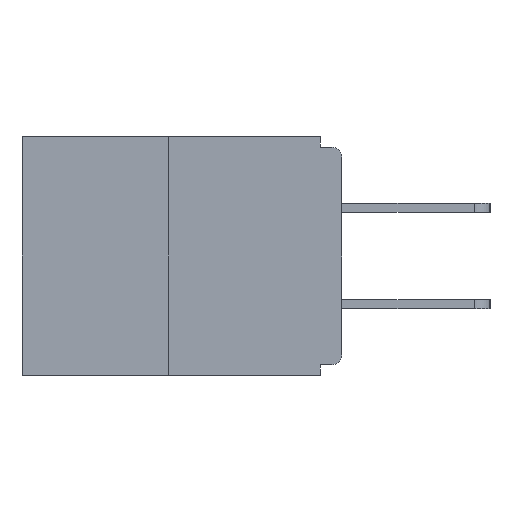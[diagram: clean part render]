
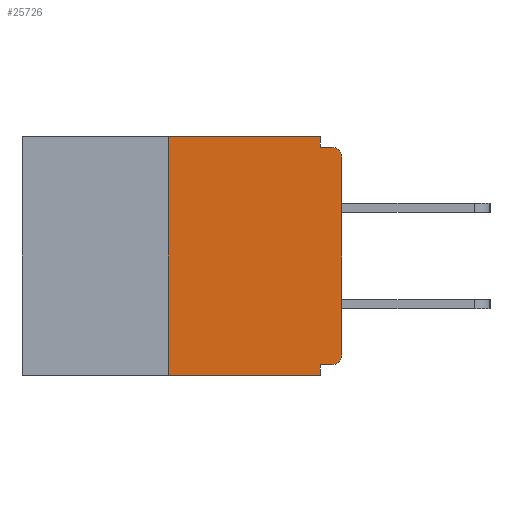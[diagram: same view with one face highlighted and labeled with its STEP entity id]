
A CAD part, left-side view. The second image highlights one B-rep face of the part: STEP entity #25726.
In plain terms, the highlighted planar face has unit normal (-1, 0, 0).
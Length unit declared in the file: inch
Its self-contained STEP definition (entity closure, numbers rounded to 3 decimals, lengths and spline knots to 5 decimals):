
#732 = VERTEX_POINT ( 'NONE', #14581 ) ;
#892 = VERTEX_POINT ( 'NONE', #1033 ) ;
#898 = EDGE_CURVE ( 'NONE', #9735, #3506, #5261, .T. ) ;
#1033 = CARTESIAN_POINT ( 'NONE',  ( 0., 0.031, -0.328 ) ) ;
#1345 = ORIENTED_EDGE ( 'NONE', *, *, #4775, .F. ) ;
#1487 = LINE ( 'NONE', #15664, #18242 ) ;
#2038 = VECTOR ( 'NONE', #20877, 39.37008 ) ;
#2136 = EDGE_CURVE ( 'NONE', #18240, #11661, #12534, .T. ) ;
#2419 = ORIENTED_EDGE ( 'NONE', *, *, #25738, .F. ) ;
#2661 = EDGE_CURVE ( 'NONE', #3296, #732, #25574, .T. ) ;
#2870 = CARTESIAN_POINT ( 'NONE',  ( 0., 0.25, 0. ) ) ;
#3296 = VERTEX_POINT ( 'NONE', #15559 ) ;
#3506 = VERTEX_POINT ( 'NONE', #11809 ) ;
#3831 = VERTEX_POINT ( 'NONE', #12158 ) ;
#4053 = ORIENTED_EDGE ( 'NONE', *, *, #15101, .T. ) ;
#4379 = DIRECTION ( 'NONE',  ( 0., 0., 1. ) ) ;
#4775 = EDGE_CURVE ( 'NONE', #892, #732, #16325, .T. ) ;
#4933 = DIRECTION ( 'NONE',  ( -1., 0., 0. ) ) ;
#5167 = FACE_OUTER_BOUND ( 'NONE', #7096, .T. ) ;
#5261 = LINE ( 'NONE', #15255, #25230 ) ;
#5532 = ORIENTED_EDGE ( 'NONE', *, *, #22705, .F. ) ;
#5595 = VECTOR ( 'NONE', #28598, 39.37008 ) ;
#5778 = CIRCLE ( 'NONE', #15363, 0.015 ) ;
#5950 = CARTESIAN_POINT ( 'NONE',  ( 0., 0., -0.03 ) ) ;
#5977 = EDGE_CURVE ( 'NONE', #11661, #3831, #5778, .T. ) ;
#5988 = ORIENTED_EDGE ( 'NONE', *, *, #2136, .T. ) ;
#6021 = VECTOR ( 'NONE', #4379, 39.37008 ) ;
#6600 = CARTESIAN_POINT ( 'NONE',  ( 0., 0.25, 0. ) ) ;
#6852 = EDGE_CURVE ( 'NONE', #3506, #3831, #20271, .T. ) ;
#6981 = CARTESIAN_POINT ( 'NONE',  ( 0., 0.46, 0. ) ) ;
#7096 = EDGE_LOOP ( 'NONE', ( #16129, #5532, #9084, #1345, #2419, #4053, #5988, #25670, #18817, #22055 ) ) ;
#9084 = ORIENTED_EDGE ( 'NONE', *, *, #2661, .T. ) ;
#9735 = VERTEX_POINT ( 'NONE', #13525 ) ;
#9974 = VECTOR ( 'NONE', #18472, 39.37008 ) ;
#10137 = VECTOR ( 'NONE', #20599, 39.37008 ) ;
#10347 = DIRECTION ( 'NONE',  ( 0., 0., 1. ) ) ;
#11661 = VERTEX_POINT ( 'NONE', #5950 ) ;
#11809 = CARTESIAN_POINT ( 'NONE',  ( 0., 0.031, -0.015 ) ) ;
#11965 = DIRECTION ( 'NONE',  ( 0., 0., -1. ) ) ;
#12128 = CARTESIAN_POINT ( 'NONE',  ( 0., 0.015, -0.328 ) ) ;
#12158 = CARTESIAN_POINT ( 'NONE',  ( 0., 0.015, -0.015 ) ) ;
#12521 = CARTESIAN_POINT ( 'NONE',  ( 0., 0., 0. ) ) ;
#12534 = LINE ( 'NONE', #12521, #17587 ) ;
#13525 = CARTESIAN_POINT ( 'NONE',  ( 0., 0.031, 0. ) ) ;
#13853 = CARTESIAN_POINT ( 'NONE',  ( 0., 0.46, 0. ) ) ;
#14177 = EDGE_CURVE ( 'NONE', #24141, #9735, #29303, .T. ) ;
#14235 = DIRECTION ( 'NONE',  ( -1., 0., 0. ) ) ;
#14581 = CARTESIAN_POINT ( 'NONE',  ( 0., 0.031, -0.343 ) ) ;
#15101 = EDGE_CURVE ( 'NONE', #27652, #18240, #16440, .T. ) ;
#15255 = CARTESIAN_POINT ( 'NONE',  ( 0., 0.031, 0. ) ) ;
#15363 = AXIS2_PLACEMENT_3D ( 'NONE', #28325, #4933, #11965 ) ;
#15559 = CARTESIAN_POINT ( 'NONE',  ( 0., 0.25, -0.343 ) ) ;
#15664 = CARTESIAN_POINT ( 'NONE',  ( 0., 0., -0.328 ) ) ;
#16129 = ORIENTED_EDGE ( 'NONE', *, *, #14177, .F. ) ;
#16325 = LINE ( 'NONE', #18434, #10137 ) ;
#16440 = CIRCLE ( 'NONE', #28398, 0.015 ) ;
#16460 = CARTESIAN_POINT ( 'NONE',  ( 0., 0., -0.313 ) ) ;
#17087 = CARTESIAN_POINT ( 'NONE',  ( 0., 0.46, -0.343 ) ) ;
#17587 = VECTOR ( 'NONE', #10347, 39.37008 ) ;
#18240 = VERTEX_POINT ( 'NONE', #16460 ) ;
#18242 = VECTOR ( 'NONE', #23023, 39.37008 ) ;
#18417 = DIRECTION ( 'NONE',  ( 1., 0., 0. ) ) ;
#18434 = CARTESIAN_POINT ( 'NONE',  ( 0., 0.031, -0.343 ) ) ;
#18472 = DIRECTION ( 'NONE',  ( 0., -1., 0. ) ) ;
#18817 = ORIENTED_EDGE ( 'NONE', *, *, #6852, .F. ) ;
#19967 = DIRECTION ( 'NONE',  ( 0., 0., -1. ) ) ;
#20271 = LINE ( 'NONE', #30146, #2038 ) ;
#20599 = DIRECTION ( 'NONE',  ( 0., 0., -1. ) ) ;
#20877 = DIRECTION ( 'NONE',  ( 0., -1., 0. ) ) ;
#22055 = ORIENTED_EDGE ( 'NONE', *, *, #898, .F. ) ;
#22705 = EDGE_CURVE ( 'NONE', #3296, #24141, #27498, .T. ) ;
#22973 = AXIS2_PLACEMENT_3D ( 'NONE', #13853, #18417, #30051 ) ;
#23023 = DIRECTION ( 'NONE',  ( 0., 1., 0. ) ) ;
#24141 = VERTEX_POINT ( 'NONE', #2870 ) ;
#25230 = VECTOR ( 'NONE', #19967, 39.37008 ) ;
#25574 = LINE ( 'NONE', #17087, #5595 ) ;
#25670 = ORIENTED_EDGE ( 'NONE', *, *, #5977, .T. ) ;
#25726 = ADVANCED_FACE ( 'NONE', ( #5167 ), #27693, .F. ) ;
#25738 = EDGE_CURVE ( 'NONE', #27652, #892, #1487, .T. ) ;
#27498 = LINE ( 'NONE', #6600, #6021 ) ;
#27652 = VERTEX_POINT ( 'NONE', #12128 ) ;
#27693 = PLANE ( 'NONE',  #22973 ) ;
#27982 = CARTESIAN_POINT ( 'NONE',  ( 0., 0.015, -0.313 ) ) ;
#28172 = DIRECTION ( 'NONE',  ( 0., 0., -1. ) ) ;
#28325 = CARTESIAN_POINT ( 'NONE',  ( 0., 0.015, -0.03 ) ) ;
#28398 = AXIS2_PLACEMENT_3D ( 'NONE', #27982, #14235, #28172 ) ;
#28598 = DIRECTION ( 'NONE',  ( 0., -1., 0. ) ) ;
#29303 = LINE ( 'NONE', #6981, #9974 ) ;
#30051 = DIRECTION ( 'NONE',  ( 0., 0., -1. ) ) ;
#30146 = CARTESIAN_POINT ( 'NONE',  ( 0., 0., -0.015 ) ) ;
